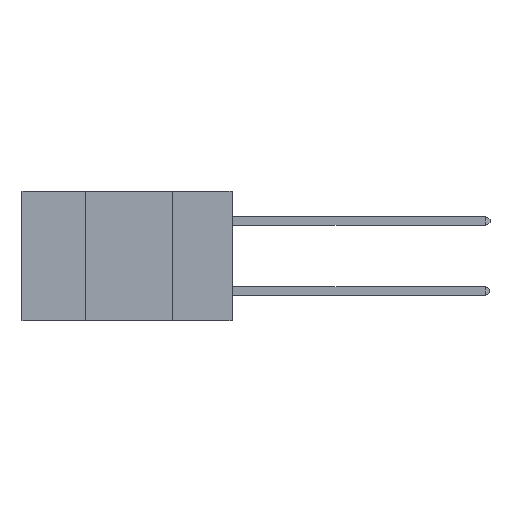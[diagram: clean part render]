
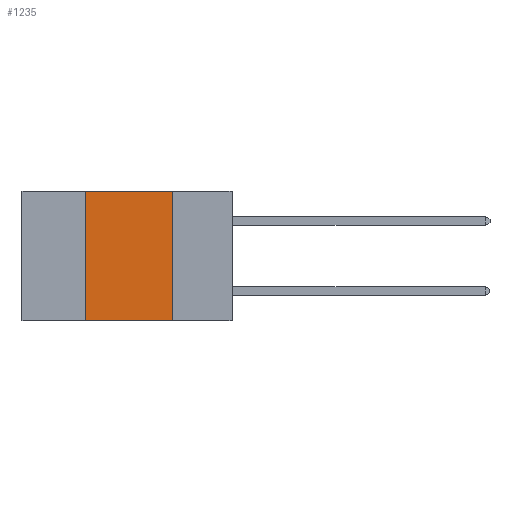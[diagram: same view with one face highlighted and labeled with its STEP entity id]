
A CAD part, left-side view. The second image highlights one B-rep face of the part: STEP entity #1235.
In plain terms, the highlighted planar face has unit normal (-1, 0, 0).
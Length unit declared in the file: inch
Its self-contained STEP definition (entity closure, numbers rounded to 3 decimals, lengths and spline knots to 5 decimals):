
#1235 = ADVANCED_FACE ( 'NONE', ( #2310 ), #1484, .F. ) ;
#1484 = PLANE ( 'NONE',  #4665 ) ;
#1492 = CARTESIAN_POINT ( 'NONE',  ( 0., 0.6, 0. ) ) ;
#2310 = FACE_OUTER_BOUND ( 'NONE', #13600, .T. ) ;
#2328 = CARTESIAN_POINT ( 'NONE',  ( 0., 0.42, 0. ) ) ;
#2465 = LINE ( 'NONE', #12607, #5774 ) ;
#2989 = VERTEX_POINT ( 'NONE', #2328 ) ;
#3379 = DIRECTION ( 'NONE',  ( 0., 0., 1. ) ) ;
#3459 = ORIENTED_EDGE ( 'NONE', *, *, #9077, .F. ) ;
#3701 = ORIENTED_EDGE ( 'NONE', *, *, #6156, .F. ) ;
#4518 = LINE ( 'NONE', #1492, #13919 ) ;
#4665 = AXIS2_PLACEMENT_3D ( 'NONE', #15333, #8749, #8713 ) ;
#5404 = VECTOR ( 'NONE', #13033, 39.37008 ) ;
#5774 = VECTOR ( 'NONE', #11369, 39.37008 ) ;
#5820 = CARTESIAN_POINT ( 'NONE',  ( 0., 0.42, 0. ) ) ;
#5993 = VECTOR ( 'NONE', #3379, 39.37008 ) ;
#6156 = EDGE_CURVE ( 'NONE', #9359, #2989, #9198, .T. ) ;
#6375 = VERTEX_POINT ( 'NONE', #12392 ) ;
#6849 = CARTESIAN_POINT ( 'NONE',  ( 0., 0.17, -0.37 ) ) ;
#6929 = CARTESIAN_POINT ( 'NONE',  ( 0., 0.17, 0. ) ) ;
#8479 = ORIENTED_EDGE ( 'NONE', *, *, #15472, .T. ) ;
#8713 = DIRECTION ( 'NONE',  ( 0., 0., -1. ) ) ;
#8749 = DIRECTION ( 'NONE',  ( 1., 0., 0. ) ) ;
#9077 = EDGE_CURVE ( 'NONE', #2989, #6375, #4518, .T. ) ;
#9198 = LINE ( 'NONE', #5820, #5993 ) ;
#9359 = VERTEX_POINT ( 'NONE', #11895 ) ;
#10121 = VERTEX_POINT ( 'NONE', #6849 ) ;
#11336 = ORIENTED_EDGE ( 'NONE', *, *, #15685, .F. ) ;
#11369 = DIRECTION ( 'NONE',  ( 0., -1., 0. ) ) ;
#11895 = CARTESIAN_POINT ( 'NONE',  ( 0., 0.42, -0.37 ) ) ;
#12392 = CARTESIAN_POINT ( 'NONE',  ( 0., 0.17, 0. ) ) ;
#12607 = CARTESIAN_POINT ( 'NONE',  ( 0., 0.6, -0.37 ) ) ;
#13033 = DIRECTION ( 'NONE',  ( 0., 0., -1. ) ) ;
#13600 = EDGE_LOOP ( 'NONE', ( #11336, #3459, #3701, #8479 ) ) ;
#13919 = VECTOR ( 'NONE', #14920, 39.37008 ) ;
#14920 = DIRECTION ( 'NONE',  ( 0., -1., 0. ) ) ;
#15333 = CARTESIAN_POINT ( 'NONE',  ( 0., 0.6, 0. ) ) ;
#15472 = EDGE_CURVE ( 'NONE', #9359, #10121, #2465, .T. ) ;
#15685 = EDGE_CURVE ( 'NONE', #6375, #10121, #15910, .T. ) ;
#15910 = LINE ( 'NONE', #6929, #5404 ) ;
